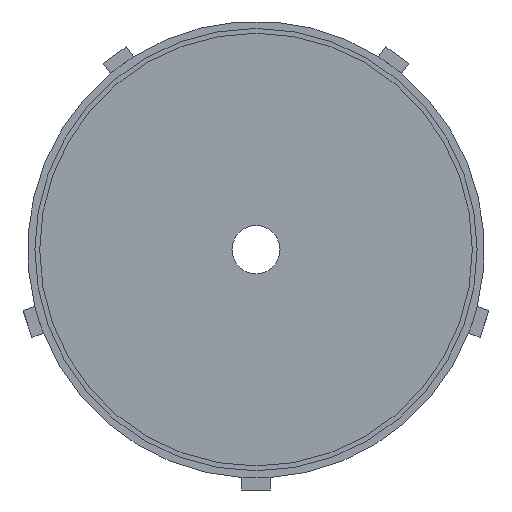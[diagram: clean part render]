
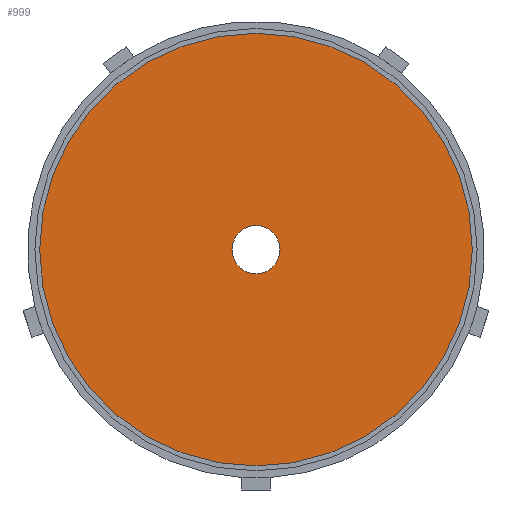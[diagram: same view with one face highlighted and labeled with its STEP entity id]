
A CAD part, front view. The second image highlights one B-rep face of the part: STEP entity #999.
In plain terms, the highlighted planar face has unit normal (0, -1, 0).
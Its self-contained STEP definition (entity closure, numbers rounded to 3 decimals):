
#14 = DIRECTION ( 'NONE',  ( 0., 0., 1. ) ) ;
#161 = DIRECTION ( 'NONE',  ( 0., -1., 0. ) ) ;
#219 = EDGE_LOOP ( 'NONE', ( #1818, #922 ) ) ;
#336 = CARTESIAN_POINT ( 'NONE',  ( 0., 70., 0. ) ) ;
#399 = CARTESIAN_POINT ( 'NONE',  ( 0., 70., 0. ) ) ;
#447 = DIRECTION ( 'NONE',  ( 0., 1., 0. ) ) ;
#564 = CARTESIAN_POINT ( 'NONE',  ( 0., 70., 0. ) ) ;
#650 = VERTEX_POINT ( 'NONE', #1715 ) ;
#681 = VERTEX_POINT ( 'NONE', #2029 ) ;
#701 = DIRECTION ( 'NONE',  ( 0., 1., 0. ) ) ;
#704 = AXIS2_PLACEMENT_3D ( 'NONE', #1018, #161, #14 ) ;
#715 = AXIS2_PLACEMENT_3D ( 'NONE', #336, #701, #1373 ) ;
#722 = CIRCLE ( 'NONE', #715, 90. ) ;
#737 = DIRECTION ( 'NONE',  ( 0., 0., 1. ) ) ;
#882 = AXIS2_PLACEMENT_3D ( 'NONE', #399, #1256, #737 ) ;
#905 = AXIS2_PLACEMENT_3D ( 'NONE', #564, #935, #1821 ) ;
#922 = ORIENTED_EDGE ( 'NONE', *, *, #1573, .F. ) ;
#935 = DIRECTION ( 'NONE',  ( 0., -1., 0. ) ) ;
#954 = CIRCLE ( 'NONE', #882, 90. ) ;
#999 = ADVANCED_FACE ( 'NONE', ( #1182, #1647 ), #1852, .F. ) ;
#1006 = CARTESIAN_POINT ( 'NONE',  ( 0., 70., -10. ) ) ;
#1012 = AXIS2_PLACEMENT_3D ( 'NONE', #1197, #447, #1646 ) ;
#1018 = CARTESIAN_POINT ( 'NONE',  ( 0., 70., 0. ) ) ;
#1132 = ORIENTED_EDGE ( 'NONE', *, *, #1347, .F. ) ;
#1177 = CIRCLE ( 'NONE', #704, 10. ) ;
#1182 = FACE_OUTER_BOUND ( 'NONE', #219, .T. ) ;
#1191 = EDGE_LOOP ( 'NONE', ( #1214, #1132 ) ) ;
#1197 = CARTESIAN_POINT ( 'NONE',  ( 0., 70., 0. ) ) ;
#1214 = ORIENTED_EDGE ( 'NONE', *, *, #1576, .F. ) ;
#1256 = DIRECTION ( 'NONE',  ( 0., 1., 0. ) ) ;
#1347 = EDGE_CURVE ( 'NONE', #1815, #1574, #1879, .T. ) ;
#1360 = EDGE_CURVE ( 'NONE', #681, #650, #954, .T. ) ;
#1373 = DIRECTION ( 'NONE',  ( 0., 0., 1. ) ) ;
#1573 = EDGE_CURVE ( 'NONE', #650, #681, #722, .T. ) ;
#1574 = VERTEX_POINT ( 'NONE', #1006 ) ;
#1576 = EDGE_CURVE ( 'NONE', #1574, #1815, #1177, .T. ) ;
#1646 = DIRECTION ( 'NONE',  ( 0., 0., 1. ) ) ;
#1647 = FACE_BOUND ( 'NONE', #1191, .T. ) ;
#1715 = CARTESIAN_POINT ( 'NONE',  ( 0., 70., 90. ) ) ;
#1815 = VERTEX_POINT ( 'NONE', #2241 ) ;
#1818 = ORIENTED_EDGE ( 'NONE', *, *, #1360, .F. ) ;
#1821 = DIRECTION ( 'NONE',  ( 0., 0., 1. ) ) ;
#1852 = PLANE ( 'NONE',  #1012 ) ;
#1879 = CIRCLE ( 'NONE', #905, 10. ) ;
#2029 = CARTESIAN_POINT ( 'NONE',  ( 0., 70., -90. ) ) ;
#2241 = CARTESIAN_POINT ( 'NONE',  ( 0., 70., 10. ) ) ;
